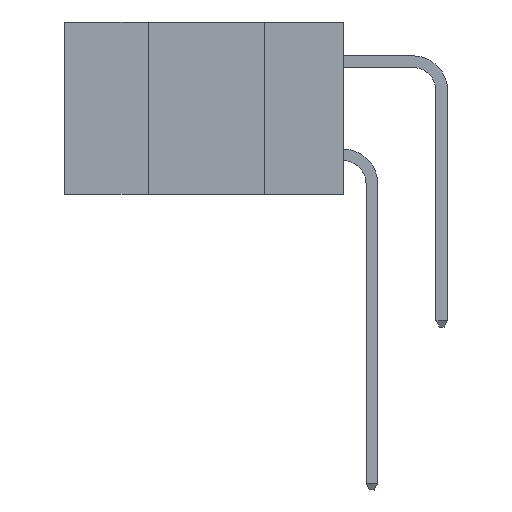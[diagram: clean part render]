
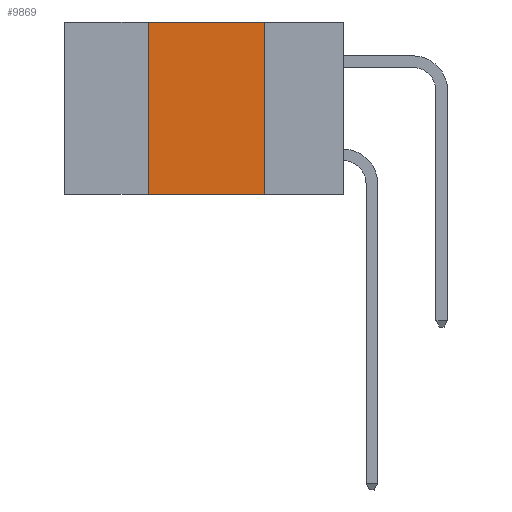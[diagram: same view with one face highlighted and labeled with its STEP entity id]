
A CAD part, left-side view. The second image highlights one B-rep face of the part: STEP entity #9869.
In plain terms, the highlighted planar face has unit normal (-1, 0, 0).
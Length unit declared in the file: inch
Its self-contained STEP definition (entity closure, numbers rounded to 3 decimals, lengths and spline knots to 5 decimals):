
#751 = DIRECTION ( 'NONE',  ( 0., -1., 0. ) ) ;
#1235 = LINE ( 'NONE', #9010, #19095 ) ;
#1333 = CARTESIAN_POINT ( 'NONE',  ( 0., 0.17, -0.37 ) ) ;
#1369 = EDGE_LOOP ( 'NONE', ( #27223, #14188, #4665, #15638 ) ) ;
#1605 = AXIS2_PLACEMENT_3D ( 'NONE', #23554, #9534, #25860 ) ;
#1615 = VECTOR ( 'NONE', #751, 39.37008 ) ;
#3049 = DIRECTION ( 'NONE',  ( 0., 0., -1. ) ) ;
#4665 = ORIENTED_EDGE ( 'NONE', *, *, #27380, .F. ) ;
#5852 = CARTESIAN_POINT ( 'NONE',  ( 0., 0.17, 0. ) ) ;
#7189 = PLANE ( 'NONE',  #1605 ) ;
#7867 = VERTEX_POINT ( 'NONE', #19194 ) ;
#8922 = DIRECTION ( 'NONE',  ( 0., 0., 1. ) ) ;
#9010 = CARTESIAN_POINT ( 'NONE',  ( 0., 0.6, 0. ) ) ;
#9534 = DIRECTION ( 'NONE',  ( 1., 0., 0. ) ) ;
#9869 = ADVANCED_FACE ( 'NONE', ( #27479 ), #7189, .F. ) ;
#11272 = EDGE_CURVE ( 'NONE', #7867, #23693, #20241, .T. ) ;
#13443 = EDGE_CURVE ( 'NONE', #19423, #23693, #26260, .T. ) ;
#14188 = ORIENTED_EDGE ( 'NONE', *, *, #21614, .F. ) ;
#15143 = LINE ( 'NONE', #22942, #27447 ) ;
#15638 = ORIENTED_EDGE ( 'NONE', *, *, #11272, .T. ) ;
#15749 = CARTESIAN_POINT ( 'NONE',  ( 0., 0.42, 0. ) ) ;
#16938 = CARTESIAN_POINT ( 'NONE',  ( 0., 0.6, -0.37 ) ) ;
#17905 = VERTEX_POINT ( 'NONE', #15749 ) ;
#18403 = DIRECTION ( 'NONE',  ( 0., -1., 0. ) ) ;
#19095 = VECTOR ( 'NONE', #18403, 39.37008 ) ;
#19194 = CARTESIAN_POINT ( 'NONE',  ( 0., 0.42, -0.37 ) ) ;
#19423 = VERTEX_POINT ( 'NONE', #5852 ) ;
#20099 = VECTOR ( 'NONE', #3049, 39.37008 ) ;
#20241 = LINE ( 'NONE', #16938, #1615 ) ;
#21614 = EDGE_CURVE ( 'NONE', #17905, #19423, #1235, .T. ) ;
#22942 = CARTESIAN_POINT ( 'NONE',  ( 0., 0.42, 0. ) ) ;
#23554 = CARTESIAN_POINT ( 'NONE',  ( 0., 0.6, 0. ) ) ;
#23693 = VERTEX_POINT ( 'NONE', #1333 ) ;
#25860 = DIRECTION ( 'NONE',  ( 0., 0., -1. ) ) ;
#26260 = LINE ( 'NONE', #28506, #20099 ) ;
#27223 = ORIENTED_EDGE ( 'NONE', *, *, #13443, .F. ) ;
#27380 = EDGE_CURVE ( 'NONE', #7867, #17905, #15143, .T. ) ;
#27447 = VECTOR ( 'NONE', #8922, 39.37008 ) ;
#27479 = FACE_OUTER_BOUND ( 'NONE', #1369, .T. ) ;
#28506 = CARTESIAN_POINT ( 'NONE',  ( 0., 0.17, 0. ) ) ;
